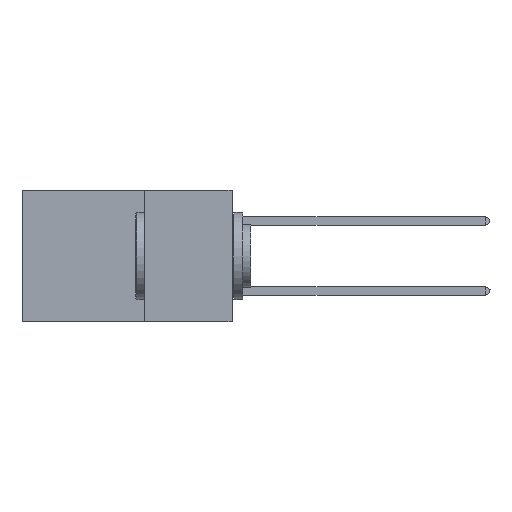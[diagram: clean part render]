
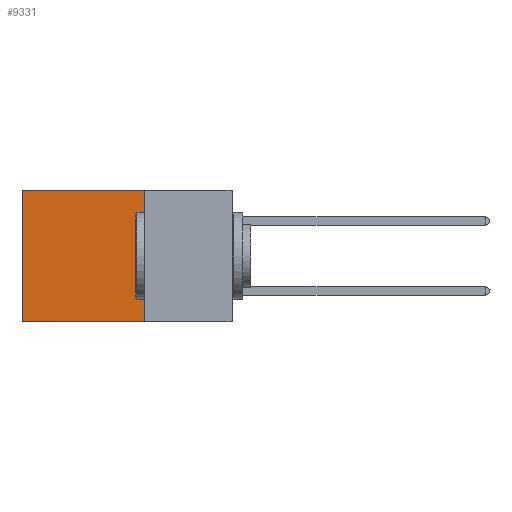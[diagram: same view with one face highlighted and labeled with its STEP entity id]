
A CAD part, left-side view. The second image highlights one B-rep face of the part: STEP entity #9331.
In plain terms, the highlighted planar face has unit normal (-1, 0, 0).
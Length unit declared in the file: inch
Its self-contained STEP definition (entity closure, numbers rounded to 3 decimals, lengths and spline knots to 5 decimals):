
#293 = CARTESIAN_POINT ( 'NONE',  ( 0.2875, 0.25, 0. ) ) ;
#604 = LINE ( 'NONE', #6348, #12878 ) ;
#751 = FACE_OUTER_BOUND ( 'NONE', #4257, .T. ) ;
#822 = CARTESIAN_POINT ( 'NONE',  ( 0.2875, 0.25, -0.375 ) ) ;
#1451 = CARTESIAN_POINT ( 'NONE',  ( 0.2875, 0.6, 0. ) ) ;
#1972 = DIRECTION ( 'NONE',  ( 0., 0., -1. ) ) ;
#2671 = LINE ( 'NONE', #822, #13054 ) ;
#4257 = EDGE_LOOP ( 'NONE', ( #17104, #15215, #11949, #7293 ) ) ;
#4391 = LINE ( 'NONE', #7921, #22402 ) ;
#4530 = AXIS2_PLACEMENT_3D ( 'NONE', #12027, #13944, #6980 ) ;
#5364 = PLANE ( 'NONE',  #4530 ) ;
#5470 = VERTEX_POINT ( 'NONE', #15986 ) ;
#6348 = CARTESIAN_POINT ( 'NONE',  ( 0.2875, 0.25, 0. ) ) ;
#6980 = DIRECTION ( 'NONE',  ( 0., 0., -1. ) ) ;
#7162 = VERTEX_POINT ( 'NONE', #8413 ) ;
#7293 = ORIENTED_EDGE ( 'NONE', *, *, #22251, .T. ) ;
#7921 = CARTESIAN_POINT ( 'NONE',  ( 0.2875, 0.6, -0.375 ) ) ;
#8413 = CARTESIAN_POINT ( 'NONE',  ( 0.2875, 0.25, -0.375 ) ) ;
#9331 = ADVANCED_FACE ( 'NONE', ( #751 ), #5364, .F. ) ;
#11949 = ORIENTED_EDGE ( 'NONE', *, *, #17292, .F. ) ;
#12027 = CARTESIAN_POINT ( 'NONE',  ( 0.2875, 0.25, -0.375 ) ) ;
#12878 = VECTOR ( 'NONE', #14891, 39.37008 ) ;
#13054 = VECTOR ( 'NONE', #14490, 39.37008 ) ;
#13944 = DIRECTION ( 'NONE',  ( 1., 0., 0. ) ) ;
#14227 = EDGE_CURVE ( 'NONE', #7162, #5470, #2671, .T. ) ;
#14490 = DIRECTION ( 'NONE',  ( 0., 1., 0. ) ) ;
#14891 = DIRECTION ( 'NONE',  ( 0., 1., 0. ) ) ;
#15215 = ORIENTED_EDGE ( 'NONE', *, *, #14227, .F. ) ;
#15986 = CARTESIAN_POINT ( 'NONE',  ( 0.2875, 0.6, -0.375 ) ) ;
#16302 = VECTOR ( 'NONE', #1972, 39.37008 ) ;
#17104 = ORIENTED_EDGE ( 'NONE', *, *, #20877, .T. ) ;
#17292 = EDGE_CURVE ( 'NONE', #17501, #7162, #18753, .T. ) ;
#17501 = VERTEX_POINT ( 'NONE', #293 ) ;
#18228 = DIRECTION ( 'NONE',  ( 0., 0., -1. ) ) ;
#18753 = LINE ( 'NONE', #21328, #16302 ) ;
#20877 = EDGE_CURVE ( 'NONE', #21097, #5470, #4391, .T. ) ;
#21097 = VERTEX_POINT ( 'NONE', #1451 ) ;
#21328 = CARTESIAN_POINT ( 'NONE',  ( 0.2875, 0.25, -0.375 ) ) ;
#22251 = EDGE_CURVE ( 'NONE', #17501, #21097, #604, .T. ) ;
#22402 = VECTOR ( 'NONE', #18228, 39.37008 ) ;
